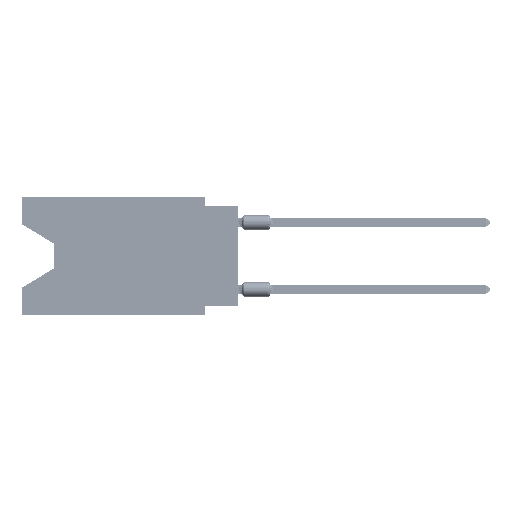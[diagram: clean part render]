
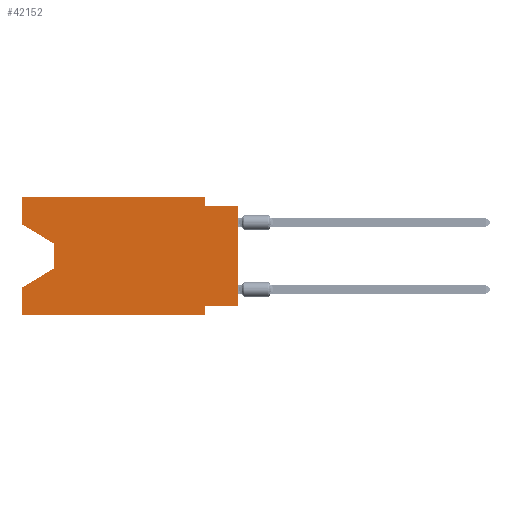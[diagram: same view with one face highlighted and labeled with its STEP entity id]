
A CAD part, left-side view. The second image highlights one B-rep face of the part: STEP entity #42152.
In plain terms, the highlighted planar face has unit normal (-1, 0, 0).
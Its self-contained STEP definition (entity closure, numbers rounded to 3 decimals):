
#220 = AXIS2_PLACEMENT_3D ( 'NONE', #10889, #36769, #63160 ) ;
#584 = ORIENTED_EDGE ( 'NONE', *, *, #28273, .F. ) ;
#715 = VERTEX_POINT ( 'NONE', #29627 ) ;
#1079 = CARTESIAN_POINT ( 'NONE',  ( 0., 13.97, -5.385 ) ) ;
#1453 = VECTOR ( 'NONE', #36863, 1000. ) ;
#4363 = ORIENTED_EDGE ( 'NONE', *, *, #16522, .F. ) ;
#4807 = VECTOR ( 'NONE', #31423, 1000. ) ;
#4931 = EDGE_CURVE ( 'NONE', #37378, #25746, #52264, .T. ) ;
#5775 = LINE ( 'NONE', #6102, #1453 ) ;
#6102 = CARTESIAN_POINT ( 'NONE',  ( 0., 2.54, -8.89 ) ) ;
#6180 = VECTOR ( 'NONE', #51722, 1000. ) ;
#6671 = ORIENTED_EDGE ( 'NONE', *, *, #4931, .T. ) ;
#7473 = CARTESIAN_POINT ( 'NONE',  ( 0., 16.383, -2.038 ) ) ;
#7527 = EDGE_CURVE ( 'NONE', #54633, #36348, #18815, .T. ) ;
#8205 = CARTESIAN_POINT ( 'NONE',  ( 0., 13.97, -5.385 ) ) ;
#9241 = ORIENTED_EDGE ( 'NONE', *, *, #45419, .T. ) ;
#10874 = VERTEX_POINT ( 'NONE', #45569 ) ;
#10889 = CARTESIAN_POINT ( 'NONE',  ( 0., 16.383, 0. ) ) ;
#11298 = ORIENTED_EDGE ( 'NONE', *, *, #29369, .F. ) ;
#11765 = CARTESIAN_POINT ( 'NONE',  ( 0., 0., -8.255 ) ) ;
#12746 = ORIENTED_EDGE ( 'NONE', *, *, #34135, .F. ) ;
#13459 = CARTESIAN_POINT ( 'NONE',  ( 0., 16.383, -2.038 ) ) ;
#15086 = VECTOR ( 'NONE', #17469, 1000. ) ;
#15722 = CARTESIAN_POINT ( 'NONE',  ( 0., 16.383, 0. ) ) ;
#16522 = EDGE_CURVE ( 'NONE', #54633, #62922, #26633, .T. ) ;
#17469 = DIRECTION ( 'NONE',  ( 0., 0., 1. ) ) ;
#17997 = EDGE_CURVE ( 'NONE', #10874, #25746, #46268, .T. ) ;
#18815 = LINE ( 'NONE', #13459, #36816 ) ;
#18970 = VECTOR ( 'NONE', #45613, 1000. ) ;
#19270 = VECTOR ( 'NONE', #65974, 1000. ) ;
#21128 = LINE ( 'NONE', #41532, #29593 ) ;
#21324 = EDGE_CURVE ( 'NONE', #54427, #59717, #46895, .T. ) ;
#21501 = CARTESIAN_POINT ( 'NONE',  ( 0., 0., 0. ) ) ;
#21723 = LINE ( 'NONE', #52822, #22604 ) ;
#22048 = EDGE_LOOP ( 'NONE', ( #56666, #9241, #30754, #12746, #42232, #65856, #11298, #6671, #49765, #584, #31894, #4363 ) ) ;
#22375 = VERTEX_POINT ( 'NONE', #24558 ) ;
#22604 = VECTOR ( 'NONE', #48129, 1000. ) ;
#22763 = CARTESIAN_POINT ( 'NONE',  ( 0., 2.54, -8.89 ) ) ;
#24558 = CARTESIAN_POINT ( 'NONE',  ( 0., 16.383, -8.89 ) ) ;
#25322 = CARTESIAN_POINT ( 'NONE',  ( 0., 16.383, 0. ) ) ;
#25348 = LINE ( 'NONE', #25678, #37553 ) ;
#25402 = EDGE_CURVE ( 'NONE', #715, #57571, #5775, .T. ) ;
#25678 = CARTESIAN_POINT ( 'NONE',  ( 0., 2.54, 0. ) ) ;
#25746 = VERTEX_POINT ( 'NONE', #36465 ) ;
#26482 = CARTESIAN_POINT ( 'NONE',  ( 0., 13.97, -3.505 ) ) ;
#26633 = LINE ( 'NONE', #25322, #6180 ) ;
#28273 = EDGE_CURVE ( 'NONE', #65233, #10874, #25348, .T. ) ;
#29054 = CARTESIAN_POINT ( 'NONE',  ( 0., 0., -8.255 ) ) ;
#29369 = EDGE_CURVE ( 'NONE', #37378, #715, #33729, .T. ) ;
#29593 = VECTOR ( 'NONE', #62240, 1000. ) ;
#29627 = CARTESIAN_POINT ( 'NONE',  ( 0., 2.54, -8.255 ) ) ;
#30754 = ORIENTED_EDGE ( 'NONE', *, *, #21324, .T. ) ;
#31423 = DIRECTION ( 'NONE',  ( 0., 0., 1. ) ) ;
#31894 = ORIENTED_EDGE ( 'NONE', *, *, #41376, .F. ) ;
#33701 = CARTESIAN_POINT ( 'NONE',  ( 0., 16.383, 0. ) ) ;
#33729 = LINE ( 'NONE', #29054, #40859 ) ;
#34135 = EDGE_CURVE ( 'NONE', #22375, #59717, #52477, .T. ) ;
#36348 = VERTEX_POINT ( 'NONE', #51747 ) ;
#36465 = CARTESIAN_POINT ( 'NONE',  ( 0., 0., -0.635 ) ) ;
#36769 = DIRECTION ( 'NONE',  ( 1., 0., 0. ) ) ;
#36816 = VECTOR ( 'NONE', #43893, 1000. ) ;
#36863 = DIRECTION ( 'NONE',  ( 0., 0., -1. ) ) ;
#37378 = VERTEX_POINT ( 'NONE', #11765 ) ;
#37553 = VECTOR ( 'NONE', #65469, 1000. ) ;
#40859 = VECTOR ( 'NONE', #49119, 1000. ) ;
#41376 = EDGE_CURVE ( 'NONE', #62922, #65233, #21723, .T. ) ;
#41532 = CARTESIAN_POINT ( 'NONE',  ( 0., 16.383, -8.89 ) ) ;
#41658 = FACE_OUTER_BOUND ( 'NONE', #22048, .T. ) ;
#42152 = ADVANCED_FACE ( 'NONE', ( #41658 ), #51687, .F. ) ;
#42232 = ORIENTED_EDGE ( 'NONE', *, *, #57431, .T. ) ;
#43893 = DIRECTION ( 'NONE',  ( 0., -0.855, -0.519 ) ) ;
#45419 = EDGE_CURVE ( 'NONE', #36348, #54427, #57896, .T. ) ;
#45569 = CARTESIAN_POINT ( 'NONE',  ( 0., 2.54, -0.635 ) ) ;
#45613 = DIRECTION ( 'NONE',  ( 0., -1., 0. ) ) ;
#46268 = LINE ( 'NONE', #61643, #18970 ) ;
#46895 = LINE ( 'NONE', #1079, #19270 ) ;
#48129 = DIRECTION ( 'NONE',  ( 0., -1., 0. ) ) ;
#48604 = VECTOR ( 'NONE', #56590, 1000. ) ;
#49119 = DIRECTION ( 'NONE',  ( 0., 1., 0. ) ) ;
#49765 = ORIENTED_EDGE ( 'NONE', *, *, #17997, .F. ) ;
#51687 = PLANE ( 'NONE',  #220 ) ;
#51722 = DIRECTION ( 'NONE',  ( 0., 0., 1. ) ) ;
#51747 = CARTESIAN_POINT ( 'NONE',  ( 0., 13.97, -3.505 ) ) ;
#52264 = LINE ( 'NONE', #21501, #15086 ) ;
#52477 = LINE ( 'NONE', #15722, #4807 ) ;
#52822 = CARTESIAN_POINT ( 'NONE',  ( 0., 16.383, 0. ) ) ;
#54038 = CARTESIAN_POINT ( 'NONE',  ( 0., 16.383, -6.852 ) ) ;
#54427 = VERTEX_POINT ( 'NONE', #8205 ) ;
#54633 = VERTEX_POINT ( 'NONE', #7473 ) ;
#56590 = DIRECTION ( 'NONE',  ( 0., 0., -1. ) ) ;
#56666 = ORIENTED_EDGE ( 'NONE', *, *, #7527, .T. ) ;
#57431 = EDGE_CURVE ( 'NONE', #22375, #57571, #21128, .T. ) ;
#57571 = VERTEX_POINT ( 'NONE', #22763 ) ;
#57896 = LINE ( 'NONE', #26482, #48604 ) ;
#59717 = VERTEX_POINT ( 'NONE', #54038 ) ;
#59901 = CARTESIAN_POINT ( 'NONE',  ( 0., 2.54, 0. ) ) ;
#61643 = CARTESIAN_POINT ( 'NONE',  ( 0., 0., -0.635 ) ) ;
#62240 = DIRECTION ( 'NONE',  ( 0., -1., 0. ) ) ;
#62922 = VERTEX_POINT ( 'NONE', #33701 ) ;
#63160 = DIRECTION ( 'NONE',  ( 0., 0., -1. ) ) ;
#65233 = VERTEX_POINT ( 'NONE', #59901 ) ;
#65469 = DIRECTION ( 'NONE',  ( 0., 0., -1. ) ) ;
#65856 = ORIENTED_EDGE ( 'NONE', *, *, #25402, .F. ) ;
#65974 = DIRECTION ( 'NONE',  ( 0., 0.855, -0.519 ) ) ;
